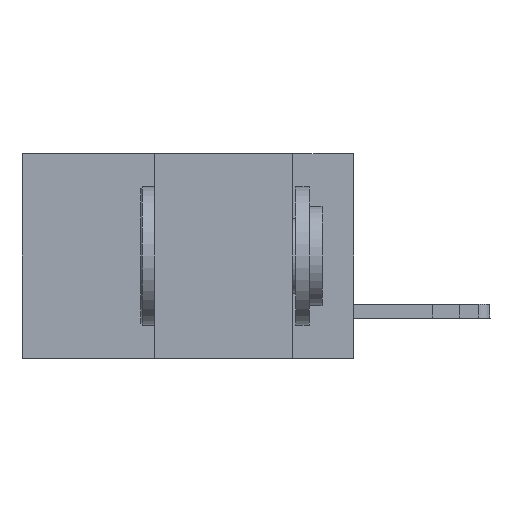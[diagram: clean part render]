
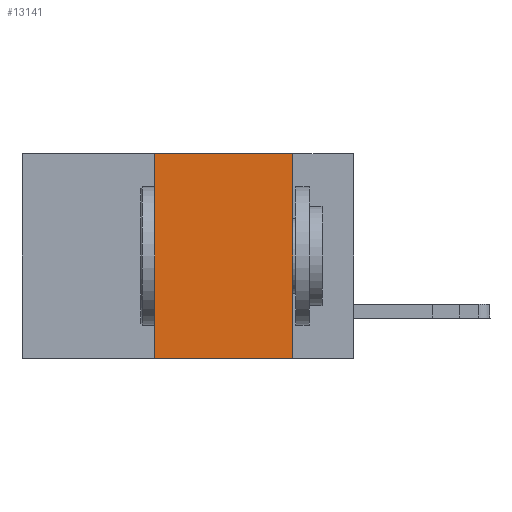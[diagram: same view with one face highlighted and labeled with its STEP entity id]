
A CAD part, left-side view. The second image highlights one B-rep face of the part: STEP entity #13141.
In plain terms, the highlighted planar face has unit normal (-1, 0, 0).
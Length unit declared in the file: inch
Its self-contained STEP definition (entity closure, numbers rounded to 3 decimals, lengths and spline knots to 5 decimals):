
#1526 = LINE ( 'NONE', #25417, #22367 ) ;
#1705 = VERTEX_POINT ( 'NONE', #1888 ) ;
#1888 = CARTESIAN_POINT ( 'NONE',  ( 0., 0.36, -0.37 ) ) ;
#1901 = DIRECTION ( 'NONE',  ( 0., -1., 0. ) ) ;
#3351 = DIRECTION ( 'NONE',  ( 0., 0., 1. ) ) ;
#3880 = DIRECTION ( 'NONE',  ( 0., -1., 0. ) ) ;
#4321 = VECTOR ( 'NONE', #1901, 39.37008 ) ;
#4335 = LINE ( 'NONE', #26050, #25179 ) ;
#4704 = AXIS2_PLACEMENT_3D ( 'NONE', #17942, #24019, #11971 ) ;
#4788 = ORIENTED_EDGE ( 'NONE', *, *, #13010, .F. ) ;
#6868 = ORIENTED_EDGE ( 'NONE', *, *, #8493, .F. ) ;
#8223 = EDGE_LOOP ( 'NONE', ( #20495, #6868, #4788, #10608 ) ) ;
#8482 = FACE_OUTER_BOUND ( 'NONE', #8223, .T. ) ;
#8493 = EDGE_CURVE ( 'NONE', #17534, #19935, #15087, .T. ) ;
#10608 = ORIENTED_EDGE ( 'NONE', *, *, #24796, .T. ) ;
#10826 = DIRECTION ( 'NONE',  ( 0., 0., -1. ) ) ;
#11876 = PLANE ( 'NONE',  #4704 ) ;
#11971 = DIRECTION ( 'NONE',  ( 0., 0., -1. ) ) ;
#12561 = LINE ( 'NONE', #22878, #23261 ) ;
#13010 = EDGE_CURVE ( 'NONE', #1705, #17534, #1526, .T. ) ;
#13141 = ADVANCED_FACE ( 'NONE', ( #8482 ), #11876, .F. ) ;
#14221 = CARTESIAN_POINT ( 'NONE',  ( 0., 0.11, -0.37 ) ) ;
#14692 = EDGE_CURVE ( 'NONE', #19935, #18282, #12561, .T. ) ;
#15087 = LINE ( 'NONE', #16042, #4321 ) ;
#16042 = CARTESIAN_POINT ( 'NONE',  ( 0., 0.6, 0. ) ) ;
#17534 = VERTEX_POINT ( 'NONE', #25680 ) ;
#17942 = CARTESIAN_POINT ( 'NONE',  ( 0., 0.6, 0. ) ) ;
#18282 = VERTEX_POINT ( 'NONE', #14221 ) ;
#19935 = VERTEX_POINT ( 'NONE', #25379 ) ;
#20495 = ORIENTED_EDGE ( 'NONE', *, *, #14692, .F. ) ;
#22367 = VECTOR ( 'NONE', #3351, 39.37008 ) ;
#22878 = CARTESIAN_POINT ( 'NONE',  ( 0., 0.11, 0. ) ) ;
#23261 = VECTOR ( 'NONE', #10826, 39.37008 ) ;
#24019 = DIRECTION ( 'NONE',  ( 1., 0., 0. ) ) ;
#24796 = EDGE_CURVE ( 'NONE', #1705, #18282, #4335, .T. ) ;
#25179 = VECTOR ( 'NONE', #3880, 39.37008 ) ;
#25379 = CARTESIAN_POINT ( 'NONE',  ( 0., 0.11, 0. ) ) ;
#25417 = CARTESIAN_POINT ( 'NONE',  ( 0., 0.36, 0. ) ) ;
#25680 = CARTESIAN_POINT ( 'NONE',  ( 0., 0.36, 0. ) ) ;
#26050 = CARTESIAN_POINT ( 'NONE',  ( 0., 0.6, -0.37 ) ) ;
